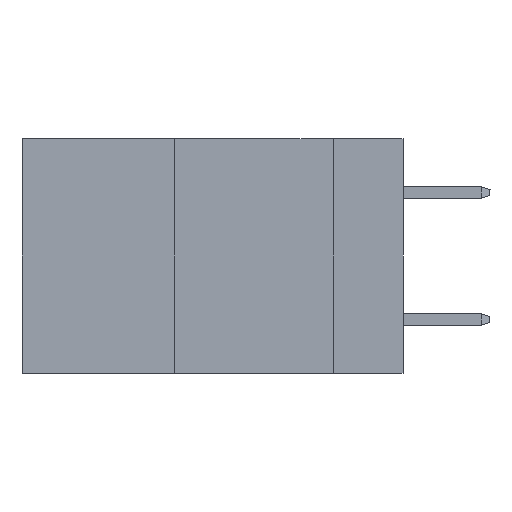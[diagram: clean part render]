
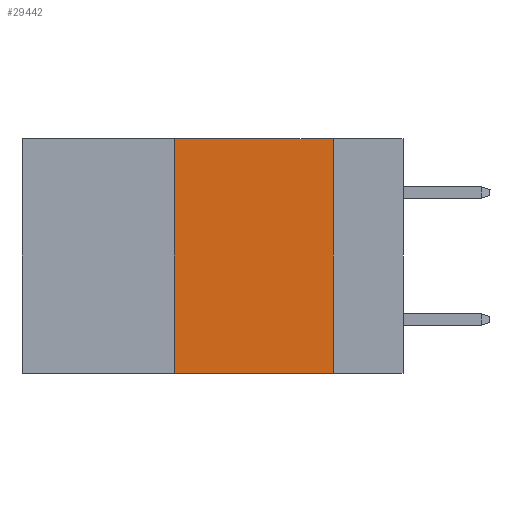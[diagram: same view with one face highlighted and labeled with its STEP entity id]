
A CAD part, left-side view. The second image highlights one B-rep face of the part: STEP entity #29442.
In plain terms, the highlighted planar face has unit normal (-1, 0, 0).
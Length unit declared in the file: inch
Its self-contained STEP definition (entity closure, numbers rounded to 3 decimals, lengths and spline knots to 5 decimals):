
#953 = CARTESIAN_POINT ( 'NONE',  ( 0., 0.6, 0. ) ) ;
#2809 = DIRECTION ( 'NONE',  ( 1., 0., 0. ) ) ;
#4813 = VERTEX_POINT ( 'NONE', #18787 ) ;
#5755 = CARTESIAN_POINT ( 'NONE',  ( 0., 0.11, 0. ) ) ;
#5918 = VERTEX_POINT ( 'NONE', #32328 ) ;
#6718 = ORIENTED_EDGE ( 'NONE', *, *, #46011, .T. ) ;
#7328 = LINE ( 'NONE', #24377, #29918 ) ;
#11570 = CARTESIAN_POINT ( 'NONE',  ( 0., 0.11, -0.37 ) ) ;
#11991 = AXIS2_PLACEMENT_3D ( 'NONE', #35654, #2809, #14224 ) ;
#12752 = EDGE_CURVE ( 'NONE', #42022, #45108, #30703, .T. ) ;
#13994 = FACE_OUTER_BOUND ( 'NONE', #33169, .T. ) ;
#14224 = DIRECTION ( 'NONE',  ( 0., 0., -1. ) ) ;
#14979 = LINE ( 'NONE', #35703, #45891 ) ;
#15173 = DIRECTION ( 'NONE',  ( 0., -1., 0. ) ) ;
#17766 = VECTOR ( 'NONE', #44958, 39.37008 ) ;
#18687 = LINE ( 'NONE', #953, #32492 ) ;
#18787 = CARTESIAN_POINT ( 'NONE',  ( 0., 0.36, 0. ) ) ;
#24377 = CARTESIAN_POINT ( 'NONE',  ( 0., 0.36, 0. ) ) ;
#28442 = PLANE ( 'NONE',  #11991 ) ;
#29442 = ADVANCED_FACE ( 'NONE', ( #13994 ), #28442, .F. ) ;
#29918 = VECTOR ( 'NONE', #42336, 39.37008 ) ;
#30382 = EDGE_CURVE ( 'NONE', #5918, #4813, #7328, .T. ) ;
#30452 = CARTESIAN_POINT ( 'NONE',  ( 0., 0.11, 0. ) ) ;
#30653 = ORIENTED_EDGE ( 'NONE', *, *, #12752, .F. ) ;
#30703 = LINE ( 'NONE', #5755, #17766 ) ;
#32328 = CARTESIAN_POINT ( 'NONE',  ( 0., 0.36, -0.37 ) ) ;
#32492 = VECTOR ( 'NONE', #15173, 39.37008 ) ;
#33169 = EDGE_LOOP ( 'NONE', ( #30653, #37360, #40586, #6718 ) ) ;
#35654 = CARTESIAN_POINT ( 'NONE',  ( 0., 0.6, 0. ) ) ;
#35703 = CARTESIAN_POINT ( 'NONE',  ( 0., 0.6, -0.37 ) ) ;
#37360 = ORIENTED_EDGE ( 'NONE', *, *, #37457, .F. ) ;
#37457 = EDGE_CURVE ( 'NONE', #4813, #42022, #18687, .T. ) ;
#39447 = DIRECTION ( 'NONE',  ( 0., -1., 0. ) ) ;
#40586 = ORIENTED_EDGE ( 'NONE', *, *, #30382, .F. ) ;
#42022 = VERTEX_POINT ( 'NONE', #30452 ) ;
#42336 = DIRECTION ( 'NONE',  ( 0., 0., 1. ) ) ;
#44958 = DIRECTION ( 'NONE',  ( 0., 0., -1. ) ) ;
#45108 = VERTEX_POINT ( 'NONE', #11570 ) ;
#45891 = VECTOR ( 'NONE', #39447, 39.37008 ) ;
#46011 = EDGE_CURVE ( 'NONE', #5918, #45108, #14979, .T. ) ;
